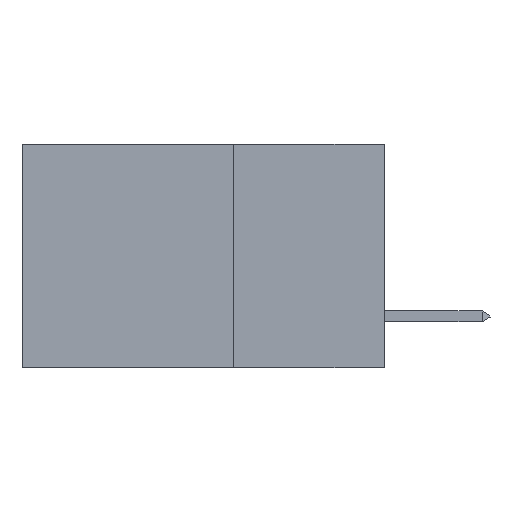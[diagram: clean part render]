
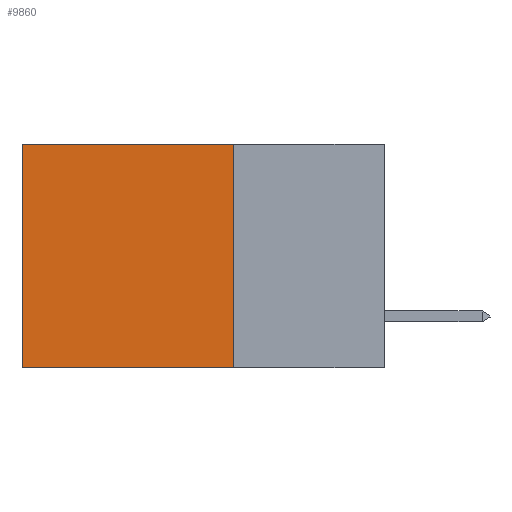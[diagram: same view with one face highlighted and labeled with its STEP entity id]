
A CAD part, left-side view. The second image highlights one B-rep face of the part: STEP entity #9860.
In plain terms, the highlighted planar face has unit normal (-1, 0, 0).
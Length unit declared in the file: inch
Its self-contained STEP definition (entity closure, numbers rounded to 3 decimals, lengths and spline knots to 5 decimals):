
#778 = EDGE_CURVE ( 'NONE', #21512, #3686, #20616, .T. ) ;
#1112 = EDGE_CURVE ( 'NONE', #21512, #15902, #11982, .T. ) ;
#2047 = DIRECTION ( 'NONE',  ( 0., 0., -1. ) ) ;
#2486 = ORIENTED_EDGE ( 'NONE', *, *, #1112, .F. ) ;
#2807 = AXIS2_PLACEMENT_3D ( 'NONE', #10283, #20466, #8282 ) ;
#3686 = VERTEX_POINT ( 'NONE', #24621 ) ;
#5523 = VECTOR ( 'NONE', #10499, 39.37008 ) ;
#7954 = ORIENTED_EDGE ( 'NONE', *, *, #778, .T. ) ;
#8239 = LINE ( 'NONE', #27167, #20821 ) ;
#8282 = DIRECTION ( 'NONE',  ( 0., 0., -1. ) ) ;
#9712 = CARTESIAN_POINT ( 'NONE',  ( 0.2875, 0.6, 0. ) ) ;
#9860 = ADVANCED_FACE ( 'NONE', ( #11537 ), #13086, .F. ) ;
#10254 = VECTOR ( 'NONE', #24049, 39.37008 ) ;
#10274 = CARTESIAN_POINT ( 'NONE',  ( 0.2875, 0.6, -0.37 ) ) ;
#10283 = CARTESIAN_POINT ( 'NONE',  ( 0.2875, 0.25, 0. ) ) ;
#10499 = DIRECTION ( 'NONE',  ( 0., 0., -1. ) ) ;
#11537 = FACE_OUTER_BOUND ( 'NONE', #15219, .T. ) ;
#11982 = LINE ( 'NONE', #20565, #5523 ) ;
#13086 = PLANE ( 'NONE',  #2807 ) ;
#14442 = CARTESIAN_POINT ( 'NONE',  ( 0.2875, 0.25, 0. ) ) ;
#15219 = EDGE_LOOP ( 'NONE', ( #17817, #22873, #2486, #7954 ) ) ;
#15902 = VERTEX_POINT ( 'NONE', #23493 ) ;
#17817 = ORIENTED_EDGE ( 'NONE', *, *, #22806, .T. ) ;
#20466 = DIRECTION ( 'NONE',  ( 1., 0., 0. ) ) ;
#20565 = CARTESIAN_POINT ( 'NONE',  ( 0.2875, 0.25, 0. ) ) ;
#20616 = LINE ( 'NONE', #14442, #10254 ) ;
#20821 = VECTOR ( 'NONE', #24707, 39.37008 ) ;
#21229 = VERTEX_POINT ( 'NONE', #10274 ) ;
#21239 = VECTOR ( 'NONE', #2047, 39.37008 ) ;
#21512 = VERTEX_POINT ( 'NONE', #31553 ) ;
#22806 = EDGE_CURVE ( 'NONE', #3686, #21229, #26601, .T. ) ;
#22873 = ORIENTED_EDGE ( 'NONE', *, *, #23456, .F. ) ;
#23456 = EDGE_CURVE ( 'NONE', #15902, #21229, #8239, .T. ) ;
#23493 = CARTESIAN_POINT ( 'NONE',  ( 0.2875, 0.25, -0.37 ) ) ;
#24049 = DIRECTION ( 'NONE',  ( 0., 1., 0. ) ) ;
#24621 = CARTESIAN_POINT ( 'NONE',  ( 0.2875, 0.6, 0. ) ) ;
#24707 = DIRECTION ( 'NONE',  ( 0., 1., 0. ) ) ;
#26601 = LINE ( 'NONE', #9712, #21239 ) ;
#27167 = CARTESIAN_POINT ( 'NONE',  ( 0.2875, 0.25, -0.37 ) ) ;
#31553 = CARTESIAN_POINT ( 'NONE',  ( 0.2875, 0.25, 0. ) ) ;
